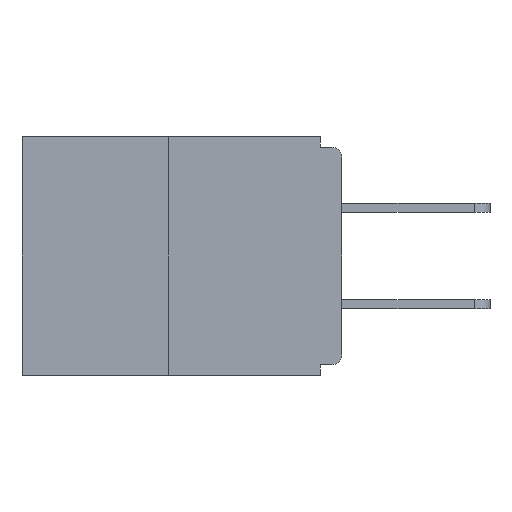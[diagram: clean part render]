
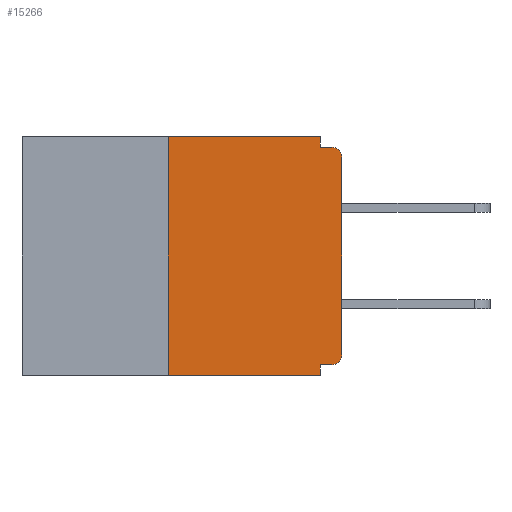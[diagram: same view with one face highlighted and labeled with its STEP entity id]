
A CAD part, left-side view. The second image highlights one B-rep face of the part: STEP entity #15266.
In plain terms, the highlighted planar face has unit normal (-1, 0, 0).
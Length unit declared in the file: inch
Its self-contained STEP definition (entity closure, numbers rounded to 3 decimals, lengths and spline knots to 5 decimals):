
#270 = VERTEX_POINT ( 'NONE', #13434 ) ;
#372 = CARTESIAN_POINT ( 'NONE',  ( 0., 0.25, -0.343 ) ) ;
#400 = CARTESIAN_POINT ( 'NONE',  ( 0., 0., 0. ) ) ;
#558 = ORIENTED_EDGE ( 'NONE', *, *, #17750, .T. ) ;
#750 = DIRECTION ( 'NONE',  ( 0., 0., 1. ) ) ;
#838 = CIRCLE ( 'NONE', #3646, 0.015 ) ;
#962 = CARTESIAN_POINT ( 'NONE',  ( 0., 0.46, -0.343 ) ) ;
#1633 = ORIENTED_EDGE ( 'NONE', *, *, #11483, .F. ) ;
#2168 = VERTEX_POINT ( 'NONE', #4114 ) ;
#2543 = DIRECTION ( 'NONE',  ( -1., 0., 0. ) ) ;
#2559 = AXIS2_PLACEMENT_3D ( 'NONE', #2803, #15954, #9379 ) ;
#2781 = DIRECTION ( 'NONE',  ( 0., -1., 0. ) ) ;
#2803 = CARTESIAN_POINT ( 'NONE',  ( 0., 0.015, -0.03 ) ) ;
#3096 = LINE ( 'NONE', #11794, #12836 ) ;
#3646 = AXIS2_PLACEMENT_3D ( 'NONE', #10777, #2543, #12861 ) ;
#4044 = CARTESIAN_POINT ( 'NONE',  ( 0., 0., -0.015 ) ) ;
#4114 = CARTESIAN_POINT ( 'NONE',  ( 0., 0.031, -0.015 ) ) ;
#4730 = LINE ( 'NONE', #17012, #12927 ) ;
#4739 = CARTESIAN_POINT ( 'NONE',  ( 0., 0.015, -0.328 ) ) ;
#4794 = EDGE_CURVE ( 'NONE', #2168, #16562, #10218, .T. ) ;
#5016 = EDGE_LOOP ( 'NONE', ( #16269, #18822, #11935, #21328, #1633, #558, #5702, #21172, #7909, #6558 ) ) ;
#5050 = EDGE_CURVE ( 'NONE', #6296, #16562, #16161, .T. ) ;
#5165 = DIRECTION ( 'NONE',  ( 0., 0., 1. ) ) ;
#5293 = LINE ( 'NONE', #400, #15079 ) ;
#5522 = LINE ( 'NONE', #11060, #12179 ) ;
#5664 = AXIS2_PLACEMENT_3D ( 'NONE', #6226, #19413, #14203 ) ;
#5702 = ORIENTED_EDGE ( 'NONE', *, *, #9989, .T. ) ;
#5712 = EDGE_CURVE ( 'NONE', #18369, #5971, #14843, .T. ) ;
#5971 = VERTEX_POINT ( 'NONE', #10593 ) ;
#6137 = VECTOR ( 'NONE', #18652, 39.37008 ) ;
#6226 = CARTESIAN_POINT ( 'NONE',  ( 0., 0.46, 0. ) ) ;
#6296 = VERTEX_POINT ( 'NONE', #19821 ) ;
#6558 = ORIENTED_EDGE ( 'NONE', *, *, #14853, .F. ) ;
#7761 = EDGE_CURVE ( 'NONE', #270, #5971, #5522, .T. ) ;
#7909 = ORIENTED_EDGE ( 'NONE', *, *, #4794, .F. ) ;
#8455 = CARTESIAN_POINT ( 'NONE',  ( 0., 0., -0.313 ) ) ;
#8949 = VECTOR ( 'NONE', #10165, 39.37008 ) ;
#9379 = DIRECTION ( 'NONE',  ( 0., 0., -1. ) ) ;
#9601 = DIRECTION ( 'NONE',  ( 0., 1., 0. ) ) ;
#9962 = LINE ( 'NONE', #13132, #8949 ) ;
#9989 = EDGE_CURVE ( 'NONE', #14889, #6296, #5293, .T. ) ;
#10165 = DIRECTION ( 'NONE',  ( 0., 0., -1. ) ) ;
#10218 = LINE ( 'NONE', #4044, #6137 ) ;
#10593 = CARTESIAN_POINT ( 'NONE',  ( 0., 0.031, -0.343 ) ) ;
#10777 = CARTESIAN_POINT ( 'NONE',  ( 0., 0.015, -0.313 ) ) ;
#11060 = CARTESIAN_POINT ( 'NONE',  ( 0., 0.031, -0.343 ) ) ;
#11099 = VERTEX_POINT ( 'NONE', #18358 ) ;
#11106 = PLANE ( 'NONE',  #5664 ) ;
#11429 = VERTEX_POINT ( 'NONE', #4739 ) ;
#11483 = EDGE_CURVE ( 'NONE', #11429, #270, #19140, .T. ) ;
#11794 = CARTESIAN_POINT ( 'NONE',  ( 0., 0.46, 0. ) ) ;
#11935 = ORIENTED_EDGE ( 'NONE', *, *, #5712, .T. ) ;
#12179 = VECTOR ( 'NONE', #20998, 39.37008 ) ;
#12836 = VECTOR ( 'NONE', #18254, 39.37008 ) ;
#12861 = DIRECTION ( 'NONE',  ( 0., 0., -1. ) ) ;
#12926 = VERTEX_POINT ( 'NONE', #15931 ) ;
#12927 = VECTOR ( 'NONE', #750, 39.37008 ) ;
#13132 = CARTESIAN_POINT ( 'NONE',  ( 0., 0.031, 0. ) ) ;
#13434 = CARTESIAN_POINT ( 'NONE',  ( 0., 0.031, -0.328 ) ) ;
#14009 = EDGE_CURVE ( 'NONE', #11099, #12926, #3096, .T. ) ;
#14203 = DIRECTION ( 'NONE',  ( 0., 0., -1. ) ) ;
#14843 = LINE ( 'NONE', #962, #17953 ) ;
#14853 = EDGE_CURVE ( 'NONE', #12926, #2168, #9962, .T. ) ;
#14889 = VERTEX_POINT ( 'NONE', #8455 ) ;
#14998 = VECTOR ( 'NONE', #9601, 39.37008 ) ;
#15079 = VECTOR ( 'NONE', #5165, 39.37008 ) ;
#15266 = ADVANCED_FACE ( 'NONE', ( #15391 ), #11106, .F. ) ;
#15391 = FACE_OUTER_BOUND ( 'NONE', #5016, .T. ) ;
#15931 = CARTESIAN_POINT ( 'NONE',  ( 0., 0.031, 0. ) ) ;
#15954 = DIRECTION ( 'NONE',  ( -1., 0., 0. ) ) ;
#16161 = CIRCLE ( 'NONE', #2559, 0.015 ) ;
#16269 = ORIENTED_EDGE ( 'NONE', *, *, #14009, .F. ) ;
#16562 = VERTEX_POINT ( 'NONE', #18792 ) ;
#17012 = CARTESIAN_POINT ( 'NONE',  ( 0., 0.25, 0. ) ) ;
#17477 = EDGE_CURVE ( 'NONE', #18369, #11099, #4730, .T. ) ;
#17750 = EDGE_CURVE ( 'NONE', #11429, #14889, #838, .T. ) ;
#17953 = VECTOR ( 'NONE', #2781, 39.37008 ) ;
#18254 = DIRECTION ( 'NONE',  ( 0., -1., 0. ) ) ;
#18358 = CARTESIAN_POINT ( 'NONE',  ( 0., 0.25, 0. ) ) ;
#18369 = VERTEX_POINT ( 'NONE', #372 ) ;
#18652 = DIRECTION ( 'NONE',  ( 0., -1., 0. ) ) ;
#18792 = CARTESIAN_POINT ( 'NONE',  ( 0., 0.015, -0.015 ) ) ;
#18822 = ORIENTED_EDGE ( 'NONE', *, *, #17477, .F. ) ;
#19140 = LINE ( 'NONE', #19561, #14998 ) ;
#19413 = DIRECTION ( 'NONE',  ( 1., 0., 0. ) ) ;
#19561 = CARTESIAN_POINT ( 'NONE',  ( 0., 0., -0.328 ) ) ;
#19821 = CARTESIAN_POINT ( 'NONE',  ( 0., 0., -0.03 ) ) ;
#20998 = DIRECTION ( 'NONE',  ( 0., 0., -1. ) ) ;
#21172 = ORIENTED_EDGE ( 'NONE', *, *, #5050, .T. ) ;
#21328 = ORIENTED_EDGE ( 'NONE', *, *, #7761, .F. ) ;
